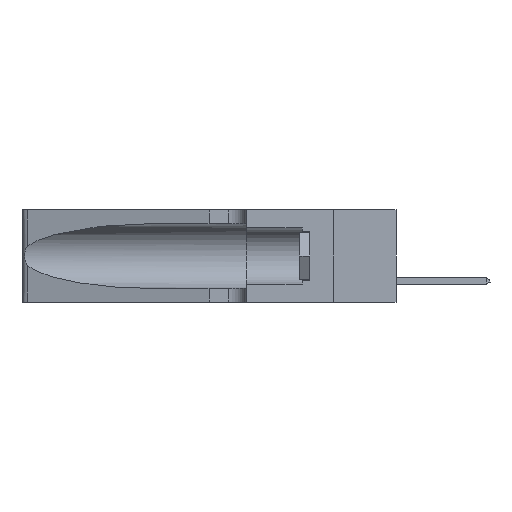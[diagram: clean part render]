
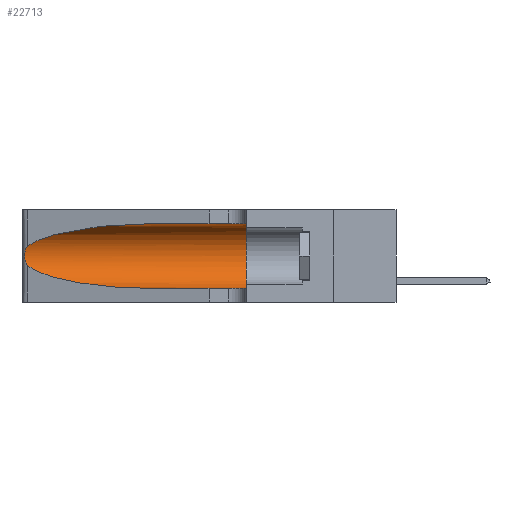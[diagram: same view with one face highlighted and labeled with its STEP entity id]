
A CAD part, left-side view. The second image highlights one B-rep face of the part: STEP entity #22713.
In plain terms, the highlighted cylindrical face has radius 3.308 mm (diameter 6.617 mm), a partial arc.
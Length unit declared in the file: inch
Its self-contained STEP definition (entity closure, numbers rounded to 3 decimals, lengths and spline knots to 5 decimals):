
#790 = CARTESIAN_POINT ( 'NONE',  ( 0.25487, 1.22718, 0.22369 ) ) ;
#1310 = DIRECTION ( 'NONE',  ( 0., 0., 1. ) ) ;
#1414 = DIRECTION ( 'NONE',  ( 0., -1., 0. ) ) ;
#1479 = CARTESIAN_POINT ( 'NONE',  ( 0.25787, 1.23484, 0.2124 ) ) ;
#1636 = ORIENTED_EDGE ( 'NONE', *, *, #21083, .T. ) ;
#1903 = EDGE_CURVE ( 'NONE', #14529, #26623, #21562, .T. ) ;
#3020 = VERTEX_POINT ( 'NONE', #14597 ) ;
#3084 = EDGE_CURVE ( 'NONE', #26623, #18180, #11614, .T. ) ;
#4071 = CARTESIAN_POINT ( 'NONE',  ( 0.25487, 1.22718, 0.14631 ) ) ;
#4635 = DIRECTION ( 'NONE',  ( 0., -1., 0. ) ) ;
#4815 = AXIS2_PLACEMENT_3D ( 'NONE', #14604, #8249, #10309 ) ;
#5480 = CARTESIAN_POINT ( 'NONE',  ( 0.26075, 1.23896, 0.19203 ) ) ;
#5499 = DIRECTION ( 'NONE',  ( 0., 1., 0. ) ) ;
#6028 = CARTESIAN_POINT ( 'NONE',  ( 0.26075, 1.23896, 0.178 ) ) ;
#7106 = LINE ( 'NONE', #10191, #15121 ) ;
#7155 = CARTESIAN_POINT ( 'NONE',  ( 0.25555, 1.22994, 0.2215 ) ) ;
#7317 =( BOUNDED_CURVE ( )  B_SPLINE_CURVE ( 3, ( #11024, #25990, #7480, #790 ),
 .UNSPECIFIED., .F., .F. ) 
 B_SPLINE_CURVE_WITH_KNOTS ( ( 4, 4 ),
 ( 1.5708, 2.84003 ),
 .UNSPECIFIED. ) 
 CURVE ( )  GEOMETRIC_REPRESENTATION_ITEM ( )  RATIONAL_B_SPLINE_CURVE ( ( 1., 0.87, 0.87, 1. ) ) 
 REPRESENTATION_ITEM ( '' )  );
#7480 = CARTESIAN_POINT ( 'NONE',  ( 0.2373, 1.15595, 0.28018 ) ) ;
#8249 = DIRECTION ( 'NONE',  ( 0., -1., 0. ) ) ;
#8686 = VECTOR ( 'NONE', #4635, 39.37008 ) ;
#9859 = CARTESIAN_POINT ( 'NONE',  ( 0.26018, 1.23835, 0.19895 ) ) ;
#10191 = CARTESIAN_POINT ( 'NONE',  ( 0.1305, 1.61858, 0.31525 ) ) ;
#10242 = CARTESIAN_POINT ( 'NONE',  ( 0.26017, 1.23833, 0.17102 ) ) ;
#10309 = DIRECTION ( 'NONE',  ( 0., 0., -1. ) ) ;
#10322 = CYLINDRICAL_SURFACE ( 'NONE', #4815, 0.13025 ) ;
#10687 = CARTESIAN_POINT ( 'NONE',  ( 0.25789, 1.23486, 0.15765 ) ) ;
#10737 = VERTEX_POINT ( 'NONE', #11468 ) ;
#10801 = CARTESIAN_POINT ( 'NONE',  ( 0.2373, 1.15595, 0.08982 ) ) ;
#10946 = ORIENTED_EDGE ( 'NONE', *, *, #24460, .F. ) ;
#11024 = CARTESIAN_POINT ( 'NONE',  ( 0.1305, 0.72297, 0.31525 ) ) ;
#11468 = CARTESIAN_POINT ( 'NONE',  ( 0.1305, 0.35, 0.05475 ) ) ;
#11614 =( BOUNDED_CURVE ( )  B_SPLINE_CURVE ( 3, ( #24198, #10801, #15003, #21742 ),
 .UNSPECIFIED., .F., .T. ) 
 B_SPLINE_CURVE_WITH_KNOTS ( ( 4, 4 ),
 ( 3.44316, 4.71239 ),
 .UNSPECIFIED. ) 
 CURVE ( )  GEOMETRIC_REPRESENTATION_ITEM ( )  RATIONAL_B_SPLINE_CURVE ( ( 1., 0.87, 0.87, 1. ) ) 
 REPRESENTATION_ITEM ( '' )  );
#12114 = CARTESIAN_POINT ( 'NONE',  ( 0.1305, 0.35, 0.185 ) ) ;
#12317 = CARTESIAN_POINT ( 'NONE',  ( 0.1305, 0.72297, 0.05475 ) ) ;
#13012 = CARTESIAN_POINT ( 'NONE',  ( 0.25487, 1.22718, 0.22369 ) ) ;
#13525 = ORIENTED_EDGE ( 'NONE', *, *, #3084, .T. ) ;
#13938 = VERTEX_POINT ( 'NONE', #15943 ) ;
#14529 = VERTEX_POINT ( 'NONE', #13012 ) ;
#14597 = CARTESIAN_POINT ( 'NONE',  ( 0.1305, 0.35, 0.31525 ) ) ;
#14604 = CARTESIAN_POINT ( 'NONE',  ( 0.1305, 1.61858, 0.185 ) ) ;
#14902 = CIRCLE ( 'NONE', #27027, 0.13025 ) ;
#15003 = CARTESIAN_POINT ( 'NONE',  ( 0.18966, 0.96281, 0.05475 ) ) ;
#15121 = VECTOR ( 'NONE', #1414, 39.37008 ) ;
#15628 = EDGE_CURVE ( 'NONE', #13938, #3020, #7106, .T. ) ;
#15943 = CARTESIAN_POINT ( 'NONE',  ( 0.1305, 0.72297, 0.31525 ) ) ;
#16324 = FACE_OUTER_BOUND ( 'NONE', #26730, .T. ) ;
#16369 = LINE ( 'NONE', #19962, #8686 ) ;
#17054 = ORIENTED_EDGE ( 'NONE', *, *, #15628, .F. ) ;
#17285 = EDGE_CURVE ( 'NONE', #13938, #14529, #7317, .T. ) ;
#18082 = CARTESIAN_POINT ( 'NONE',  ( 0.25487, 1.22718, 0.22369 ) ) ;
#18180 = VERTEX_POINT ( 'NONE', #12317 ) ;
#18268 = CARTESIAN_POINT ( 'NONE',  ( 0.25854, 1.2359, 0.20912 ) ) ;
#19962 = CARTESIAN_POINT ( 'NONE',  ( 0.1305, 1.61858, 0.05475 ) ) ;
#21083 = EDGE_CURVE ( 'NONE', #18180, #10737, #16369, .T. ) ;
#21562 = B_SPLINE_CURVE_WITH_KNOTS ( 'NONE', 3,
 ( #18082, #7155, #22403, #1479, #18268, #9859, #5480, #6028, #10242, #23523, #10687, #25746, #24627, #25633 ),
 .UNSPECIFIED., .F., .F.,
 ( 4, 2, 2, 2, 2, 2, 4 ),
 ( 0., 0.00027, 0.00053, 0.00107, 0.0016, 0.00187, 0.00214 ),
 .UNSPECIFIED. ) ;
#21742 = CARTESIAN_POINT ( 'NONE',  ( 0.1305, 0.72297, 0.05475 ) ) ;
#22403 = CARTESIAN_POINT ( 'NONE',  ( 0.25639, 1.23184, 0.21858 ) ) ;
#22713 = ADVANCED_FACE ( 'NONE', ( #16324 ), #10322, .F. ) ;
#23523 = CARTESIAN_POINT ( 'NONE',  ( 0.25856, 1.23593, 0.16098 ) ) ;
#24198 = CARTESIAN_POINT ( 'NONE',  ( 0.25487, 1.22718, 0.14631 ) ) ;
#24460 = EDGE_CURVE ( 'NONE', #3020, #10737, #14902, .T. ) ;
#24627 = CARTESIAN_POINT ( 'NONE',  ( 0.25555, 1.22993, 0.14849 ) ) ;
#25633 = CARTESIAN_POINT ( 'NONE',  ( 0.25487, 1.22718, 0.14631 ) ) ;
#25746 = CARTESIAN_POINT ( 'NONE',  ( 0.25639, 1.23186, 0.15144 ) ) ;
#25990 = CARTESIAN_POINT ( 'NONE',  ( 0.18966, 0.96281, 0.31525 ) ) ;
#26565 = ORIENTED_EDGE ( 'NONE', *, *, #17285, .T. ) ;
#26623 = VERTEX_POINT ( 'NONE', #4071 ) ;
#26730 = EDGE_LOOP ( 'NONE', ( #26565, #27268, #13525, #1636, #10946, #17054 ) ) ;
#27027 = AXIS2_PLACEMENT_3D ( 'NONE', #12114, #5499, #1310 ) ;
#27268 = ORIENTED_EDGE ( 'NONE', *, *, #1903, .T. ) ;
